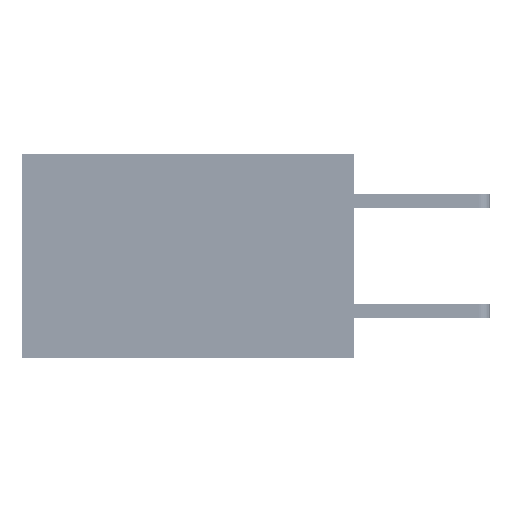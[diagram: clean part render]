
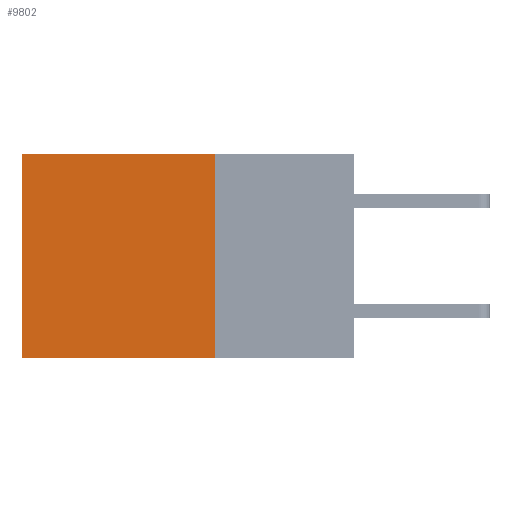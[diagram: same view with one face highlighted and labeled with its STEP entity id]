
A CAD part, left-side view. The second image highlights one B-rep face of the part: STEP entity #9802.
In plain terms, the highlighted planar face has unit normal (-1, 0, 0).
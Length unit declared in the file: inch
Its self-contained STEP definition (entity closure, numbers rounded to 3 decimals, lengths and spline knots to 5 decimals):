
#1059 = LINE ( 'NONE', #36839, #39868 ) ;
#1283 = CARTESIAN_POINT ( 'NONE',  ( 0.2875, 0.25, 0. ) ) ;
#1667 = ORIENTED_EDGE ( 'NONE', *, *, #15964, .T. ) ;
#5042 = LINE ( 'NONE', #36286, #12650 ) ;
#5880 = EDGE_LOOP ( 'NONE', ( #36703, #32967, #29840, #1667 ) ) ;
#6754 = EDGE_CURVE ( 'NONE', #18930, #25138, #27318, .T. ) ;
#6912 = DIRECTION ( 'NONE',  ( 1., 0., 0. ) ) ;
#7119 = FACE_OUTER_BOUND ( 'NONE', #5880, .T. ) ;
#8366 = DIRECTION ( 'NONE',  ( 0., 0., -1. ) ) ;
#8526 = EDGE_CURVE ( 'NONE', #25138, #36500, #21416, .T. ) ;
#9802 = ADVANCED_FACE ( 'NONE', ( #7119 ), #35453, .F. ) ;
#10582 = VERTEX_POINT ( 'NONE', #29675 ) ;
#12650 = VECTOR ( 'NONE', #26706, 39.37008 ) ;
#12984 = AXIS2_PLACEMENT_3D ( 'NONE', #1283, #6912, #23349 ) ;
#14112 = VECTOR ( 'NONE', #8366, 39.37008 ) ;
#15152 = DIRECTION ( 'NONE',  ( 0., 1., 0. ) ) ;
#15964 = EDGE_CURVE ( 'NONE', #18930, #10582, #1059, .T. ) ;
#16255 = VECTOR ( 'NONE', #31224, 39.37008 ) ;
#18752 = CARTESIAN_POINT ( 'NONE',  ( 0.2875, 0.25, 0. ) ) ;
#18930 = VERTEX_POINT ( 'NONE', #18752 ) ;
#21416 = LINE ( 'NONE', #24131, #16255 ) ;
#23349 = DIRECTION ( 'NONE',  ( 0., 0., -1. ) ) ;
#24131 = CARTESIAN_POINT ( 'NONE',  ( 0.2875, 0.25, -0.37 ) ) ;
#25138 = VERTEX_POINT ( 'NONE', #31800 ) ;
#26706 = DIRECTION ( 'NONE',  ( 0., 0., -1. ) ) ;
#27318 = LINE ( 'NONE', #40022, #14112 ) ;
#29675 = CARTESIAN_POINT ( 'NONE',  ( 0.2875, 0.6, 0. ) ) ;
#29840 = ORIENTED_EDGE ( 'NONE', *, *, #6754, .F. ) ;
#31224 = DIRECTION ( 'NONE',  ( 0., 1., 0. ) ) ;
#31565 = CARTESIAN_POINT ( 'NONE',  ( 0.2875, 0.6, -0.37 ) ) ;
#31800 = CARTESIAN_POINT ( 'NONE',  ( 0.2875, 0.25, -0.37 ) ) ;
#32967 = ORIENTED_EDGE ( 'NONE', *, *, #8526, .F. ) ;
#35453 = PLANE ( 'NONE',  #12984 ) ;
#36286 = CARTESIAN_POINT ( 'NONE',  ( 0.2875, 0.6, 0. ) ) ;
#36500 = VERTEX_POINT ( 'NONE', #31565 ) ;
#36703 = ORIENTED_EDGE ( 'NONE', *, *, #40904, .T. ) ;
#36839 = CARTESIAN_POINT ( 'NONE',  ( 0.2875, 0.25, 0. ) ) ;
#39868 = VECTOR ( 'NONE', #15152, 39.37008 ) ;
#40022 = CARTESIAN_POINT ( 'NONE',  ( 0.2875, 0.25, 0. ) ) ;
#40904 = EDGE_CURVE ( 'NONE', #10582, #36500, #5042, .T. ) ;
